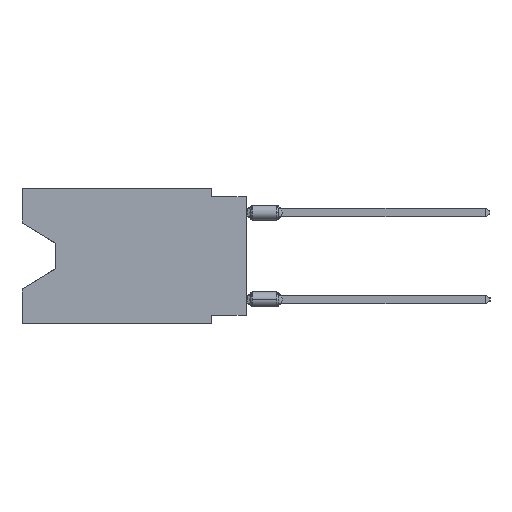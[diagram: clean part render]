
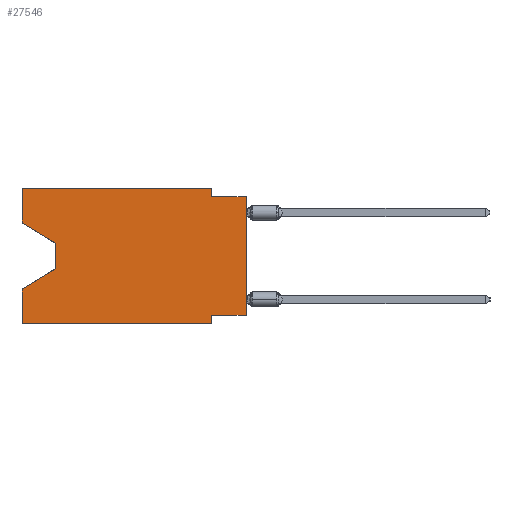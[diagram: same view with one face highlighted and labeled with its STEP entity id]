
A CAD part, left-side view. The second image highlights one B-rep face of the part: STEP entity #27546.
In plain terms, the highlighted planar face has unit normal (-1, 0, 0).
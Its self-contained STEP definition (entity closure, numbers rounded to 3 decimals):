
#62 = CARTESIAN_POINT ( 'NONE',  ( 0., 2.54, -9.906 ) ) ;
#360 = DIRECTION ( 'NONE',  ( 0., 0., 1. ) ) ;
#1036 = ORIENTED_EDGE ( 'NONE', *, *, #6781, .T. ) ;
#1319 = EDGE_LOOP ( 'NONE', ( #37662, #1036, #38909, #40757, #17997, #5658, #36369, #4341, #18125, #36528, #46574, #20984 ) ) ;
#1772 = EDGE_CURVE ( 'NONE', #29908, #46071, #21055, .T. ) ;
#1897 = CARTESIAN_POINT ( 'NONE',  ( 0., 2.54, -9.906 ) ) ;
#2118 = CARTESIAN_POINT ( 'NONE',  ( 0., 0., 0. ) ) ;
#2671 = VECTOR ( 'NONE', #10131, 1000. ) ;
#2889 = VECTOR ( 'NONE', #35417, 1000. ) ;
#2981 = LINE ( 'NONE', #39635, #22406 ) ;
#2996 = EDGE_CURVE ( 'NONE', #40521, #29908, #6079, .T. ) ;
#3576 = CARTESIAN_POINT ( 'NONE',  ( 0., 13.97, -5.893 ) ) ;
#3709 = DIRECTION ( 'NONE',  ( 1., 0., 0. ) ) ;
#3941 = DIRECTION ( 'NONE',  ( 0., 0., -1. ) ) ;
#4341 = ORIENTED_EDGE ( 'NONE', *, *, #46203, .T. ) ;
#4379 = EDGE_CURVE ( 'NONE', #14114, #29248, #23757, .T. ) ;
#4475 = CARTESIAN_POINT ( 'NONE',  ( 0., 13.97, -4.013 ) ) ;
#5053 = VERTEX_POINT ( 'NONE', #22636 ) ;
#5324 = DIRECTION ( 'NONE',  ( 0., -0.855, -0.519 ) ) ;
#5465 = VERTEX_POINT ( 'NONE', #15773 ) ;
#5658 = ORIENTED_EDGE ( 'NONE', *, *, #19242, .F. ) ;
#6079 = LINE ( 'NONE', #48030, #44490 ) ;
#6781 = EDGE_CURVE ( 'NONE', #29248, #36434, #33615, .T. ) ;
#7956 = DIRECTION ( 'NONE',  ( 0., 1., 0. ) ) ;
#8450 = LINE ( 'NONE', #45362, #34953 ) ;
#9046 = EDGE_CURVE ( 'NONE', #14114, #5053, #44324, .T. ) ;
#9407 = DIRECTION ( 'NONE',  ( 0., 0., 1. ) ) ;
#9508 = VERTEX_POINT ( 'NONE', #62 ) ;
#9601 = DIRECTION ( 'NONE',  ( 0., 0., 1. ) ) ;
#10131 = DIRECTION ( 'NONE',  ( 0., -1., 0. ) ) ;
#11295 = EDGE_CURVE ( 'NONE', #26358, #27210, #42877, .T. ) ;
#11950 = DIRECTION ( 'NONE',  ( 0., -1., 0. ) ) ;
#12090 = DIRECTION ( 'NONE',  ( 0., 0.855, -0.519 ) ) ;
#13288 = LINE ( 'NONE', #2118, #45872 ) ;
#14114 = VERTEX_POINT ( 'NONE', #29082 ) ;
#14156 = VECTOR ( 'NONE', #27035, 1000. ) ;
#15358 = FACE_OUTER_BOUND ( 'NONE', #1319, .T. ) ;
#15362 = EDGE_CURVE ( 'NONE', #5465, #45288, #44383, .T. ) ;
#15773 = CARTESIAN_POINT ( 'NONE',  ( 0., 0., -9.271 ) ) ;
#16727 = CARTESIAN_POINT ( 'NONE',  ( 0., 16.383, -2.546 ) ) ;
#17793 = DIRECTION ( 'NONE',  ( 0., -1., 0. ) ) ;
#17997 = ORIENTED_EDGE ( 'NONE', *, *, #23723, .T. ) ;
#18125 = ORIENTED_EDGE ( 'NONE', *, *, #1772, .F. ) ;
#18945 = CARTESIAN_POINT ( 'NONE',  ( 0., 2.54, -0.635 ) ) ;
#19242 = EDGE_CURVE ( 'NONE', #45288, #9508, #38336, .T. ) ;
#20210 = CARTESIAN_POINT ( 'NONE',  ( 0., 2.54, -9.271 ) ) ;
#20984 = ORIENTED_EDGE ( 'NONE', *, *, #9046, .F. ) ;
#21055 = LINE ( 'NONE', #46581, #2671 ) ;
#21221 = VECTOR ( 'NONE', #7956, 1000. ) ;
#22406 = VECTOR ( 'NONE', #17793, 1000. ) ;
#22509 = CARTESIAN_POINT ( 'NONE',  ( 0., 0., -9.271 ) ) ;
#22636 = CARTESIAN_POINT ( 'NONE',  ( 0., 16.383, 0. ) ) ;
#23088 = CARTESIAN_POINT ( 'NONE',  ( 0., 16.383, -9.906 ) ) ;
#23723 = EDGE_CURVE ( 'NONE', #26358, #9508, #2981, .T. ) ;
#23757 = LINE ( 'NONE', #16727, #26416 ) ;
#23760 = CARTESIAN_POINT ( 'NONE',  ( 0., 13.97, -4.013 ) ) ;
#25126 = EDGE_CURVE ( 'NONE', #5053, #40521, #37458, .T. ) ;
#26358 = VERTEX_POINT ( 'NONE', #23088 ) ;
#26416 = VECTOR ( 'NONE', #5324, 1000. ) ;
#27031 = CARTESIAN_POINT ( 'NONE',  ( 0., 2.54, 0. ) ) ;
#27035 = DIRECTION ( 'NONE',  ( 0., 0., -1. ) ) ;
#27210 = VERTEX_POINT ( 'NONE', #33922 ) ;
#27222 = AXIS2_PLACEMENT_3D ( 'NONE', #30170, #3709, #3941 ) ;
#27546 = ADVANCED_FACE ( 'NONE', ( #15358 ), #40613, .F. ) ;
#29082 = CARTESIAN_POINT ( 'NONE',  ( 0., 16.383, -2.546 ) ) ;
#29248 = VERTEX_POINT ( 'NONE', #23760 ) ;
#29564 = DIRECTION ( 'NONE',  ( 0., 0., -1. ) ) ;
#29908 = VERTEX_POINT ( 'NONE', #18945 ) ;
#30170 = CARTESIAN_POINT ( 'NONE',  ( 0., 16.383, 0. ) ) ;
#33615 = LINE ( 'NONE', #4475, #14156 ) ;
#33637 = EDGE_CURVE ( 'NONE', #36434, #27210, #8450, .T. ) ;
#33922 = CARTESIAN_POINT ( 'NONE',  ( 0., 16.383, -7.36 ) ) ;
#34953 = VECTOR ( 'NONE', #12090, 1000. ) ;
#35417 = DIRECTION ( 'NONE',  ( 0., 0., -1. ) ) ;
#36369 = ORIENTED_EDGE ( 'NONE', *, *, #15362, .F. ) ;
#36434 = VERTEX_POINT ( 'NONE', #3576 ) ;
#36528 = ORIENTED_EDGE ( 'NONE', *, *, #2996, .F. ) ;
#36920 = VECTOR ( 'NONE', #11950, 1000. ) ;
#37458 = LINE ( 'NONE', #45466, #36920 ) ;
#37662 = ORIENTED_EDGE ( 'NONE', *, *, #4379, .T. ) ;
#38336 = LINE ( 'NONE', #1897, #2889 ) ;
#38909 = ORIENTED_EDGE ( 'NONE', *, *, #33637, .T. ) ;
#39635 = CARTESIAN_POINT ( 'NONE',  ( 0., 16.383, -9.906 ) ) ;
#40448 = CARTESIAN_POINT ( 'NONE',  ( 0., 16.383, 0. ) ) ;
#40521 = VERTEX_POINT ( 'NONE', #27031 ) ;
#40613 = PLANE ( 'NONE',  #27222 ) ;
#40757 = ORIENTED_EDGE ( 'NONE', *, *, #11295, .F. ) ;
#42877 = LINE ( 'NONE', #45805, #43075 ) ;
#43075 = VECTOR ( 'NONE', #9601, 1000. ) ;
#44324 = LINE ( 'NONE', #40448, #46061 ) ;
#44383 = LINE ( 'NONE', #22509, #21221 ) ;
#44490 = VECTOR ( 'NONE', #29564, 1000. ) ;
#45288 = VERTEX_POINT ( 'NONE', #20210 ) ;
#45362 = CARTESIAN_POINT ( 'NONE',  ( 0., 13.97, -5.893 ) ) ;
#45466 = CARTESIAN_POINT ( 'NONE',  ( 0., 16.383, 0. ) ) ;
#45805 = CARTESIAN_POINT ( 'NONE',  ( 0., 16.383, 0. ) ) ;
#45846 = CARTESIAN_POINT ( 'NONE',  ( 0., 0., -0.635 ) ) ;
#45872 = VECTOR ( 'NONE', #9407, 1000. ) ;
#46061 = VECTOR ( 'NONE', #360, 1000. ) ;
#46071 = VERTEX_POINT ( 'NONE', #45846 ) ;
#46203 = EDGE_CURVE ( 'NONE', #5465, #46071, #13288, .T. ) ;
#46574 = ORIENTED_EDGE ( 'NONE', *, *, #25126, .F. ) ;
#46581 = CARTESIAN_POINT ( 'NONE',  ( 0., 0., -0.635 ) ) ;
#48030 = CARTESIAN_POINT ( 'NONE',  ( 0., 2.54, 0. ) ) ;
